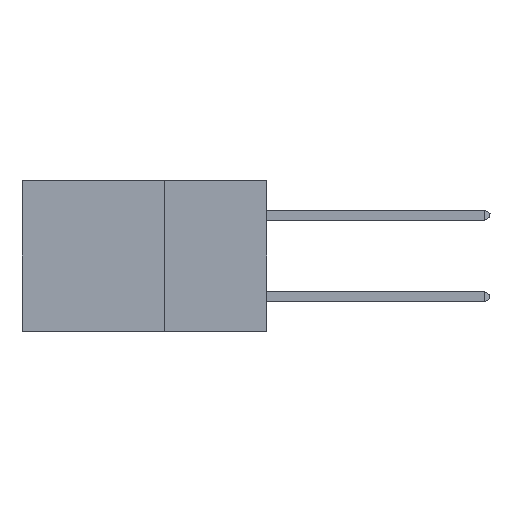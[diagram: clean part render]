
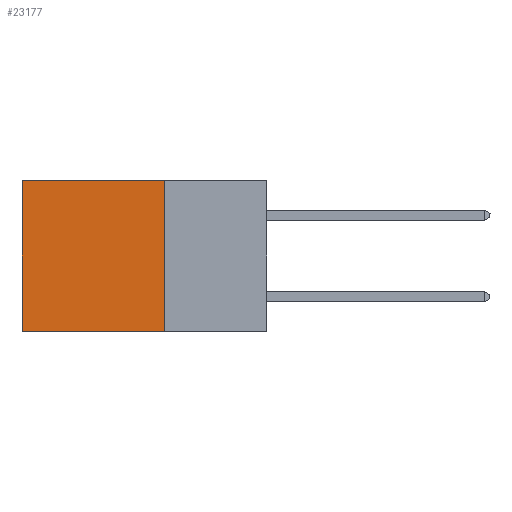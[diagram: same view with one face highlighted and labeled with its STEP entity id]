
A CAD part, left-side view. The second image highlights one B-rep face of the part: STEP entity #23177.
In plain terms, the highlighted planar face has unit normal (-1, 0, 0).
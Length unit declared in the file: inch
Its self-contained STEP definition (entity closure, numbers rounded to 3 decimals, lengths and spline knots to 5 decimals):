
#1341 = LINE ( 'NONE', #29797, #30410 ) ;
#3837 = CARTESIAN_POINT ( 'NONE',  ( 0.2875, 0.6, 0. ) ) ;
#4388 = ORIENTED_EDGE ( 'NONE', *, *, #9660, .T. ) ;
#4598 = DIRECTION ( 'NONE',  ( 0., 0., -1. ) ) ;
#4635 = DIRECTION ( 'NONE',  ( 0., 0., -1. ) ) ;
#7070 = CARTESIAN_POINT ( 'NONE',  ( 0.2875, 0.25, 0. ) ) ;
#9130 = VECTOR ( 'NONE', #15505, 39.37008 ) ;
#9407 = EDGE_CURVE ( 'NONE', #18897, #12326, #1341, .T. ) ;
#9660 = EDGE_CURVE ( 'NONE', #18897, #29914, #12891, .T. ) ;
#11461 = EDGE_LOOP ( 'NONE', ( #13312, #15130, #21552, #4388 ) ) ;
#11956 = DIRECTION ( 'NONE',  ( 1., 0., 0. ) ) ;
#12326 = VERTEX_POINT ( 'NONE', #12628 ) ;
#12628 = CARTESIAN_POINT ( 'NONE',  ( 0.2875, 0.25, -0.37 ) ) ;
#12891 = LINE ( 'NONE', #18265, #9130 ) ;
#13312 = ORIENTED_EDGE ( 'NONE', *, *, #25339, .T. ) ;
#14070 = LINE ( 'NONE', #3837, #29966 ) ;
#15082 = CARTESIAN_POINT ( 'NONE',  ( 0.2875, 0.25, 0. ) ) ;
#15130 = ORIENTED_EDGE ( 'NONE', *, *, #20693, .F. ) ;
#15505 = DIRECTION ( 'NONE',  ( 0., 1., 0. ) ) ;
#15641 = CARTESIAN_POINT ( 'NONE',  ( 0.2875, 0.25, -0.37 ) ) ;
#17182 = PLANE ( 'NONE',  #28327 ) ;
#18265 = CARTESIAN_POINT ( 'NONE',  ( 0.2875, 0.25, 0. ) ) ;
#18646 = DIRECTION ( 'NONE',  ( 0., 0., -1. ) ) ;
#18897 = VERTEX_POINT ( 'NONE', #15082 ) ;
#20051 = DIRECTION ( 'NONE',  ( 0., 1., 0. ) ) ;
#20514 = VERTEX_POINT ( 'NONE', #21667 ) ;
#20693 = EDGE_CURVE ( 'NONE', #12326, #20514, #27497, .T. ) ;
#21552 = ORIENTED_EDGE ( 'NONE', *, *, #9407, .F. ) ;
#21667 = CARTESIAN_POINT ( 'NONE',  ( 0.2875, 0.6, -0.37 ) ) ;
#21719 = FACE_OUTER_BOUND ( 'NONE', #11461, .T. ) ;
#23177 = ADVANCED_FACE ( 'NONE', ( #21719 ), #17182, .F. ) ;
#23304 = CARTESIAN_POINT ( 'NONE',  ( 0.2875, 0.6, 0. ) ) ;
#25339 = EDGE_CURVE ( 'NONE', #29914, #20514, #14070, .T. ) ;
#27497 = LINE ( 'NONE', #15641, #29840 ) ;
#28327 = AXIS2_PLACEMENT_3D ( 'NONE', #7070, #11956, #4635 ) ;
#29797 = CARTESIAN_POINT ( 'NONE',  ( 0.2875, 0.25, 0. ) ) ;
#29840 = VECTOR ( 'NONE', #20051, 39.37008 ) ;
#29914 = VERTEX_POINT ( 'NONE', #23304 ) ;
#29966 = VECTOR ( 'NONE', #18646, 39.37008 ) ;
#30410 = VECTOR ( 'NONE', #4598, 39.37008 ) ;
